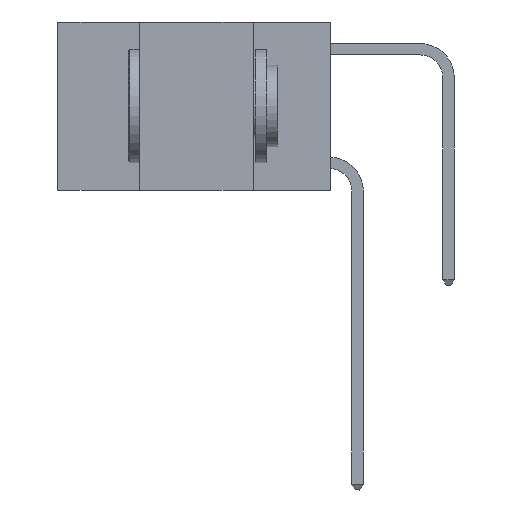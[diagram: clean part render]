
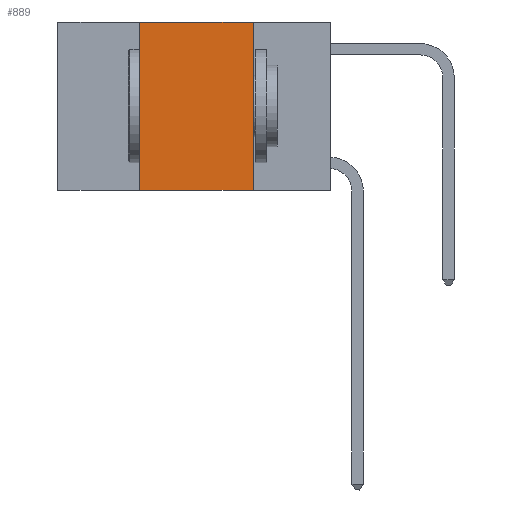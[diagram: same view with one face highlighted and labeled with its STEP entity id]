
A CAD part, left-side view. The second image highlights one B-rep face of the part: STEP entity #889.
In plain terms, the highlighted planar face has unit normal (-1, 0, 0).
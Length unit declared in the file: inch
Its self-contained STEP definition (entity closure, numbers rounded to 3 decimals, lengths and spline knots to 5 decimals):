
#241 = ORIENTED_EDGE ( 'NONE', *, *, #9986, .F. ) ;
#254 = ORIENTED_EDGE ( 'NONE', *, *, #3844, .F. ) ;
#283 = DIRECTION ( 'NONE',  ( 0., 0., 1. ) ) ;
#298 = ORIENTED_EDGE ( 'NONE', *, *, #2192, .F. ) ;
#307 = ORIENTED_EDGE ( 'NONE', *, *, #10433, .T. ) ;
#889 = ADVANCED_FACE ( 'NONE', ( #7766 ), #7281, .F. ) ;
#1146 = CARTESIAN_POINT ( 'NONE',  ( 0., 0.42, 0. ) ) ;
#1429 = VERTEX_POINT ( 'NONE', #4539 ) ;
#1534 = VERTEX_POINT ( 'NONE', #2577 ) ;
#1878 = AXIS2_PLACEMENT_3D ( 'NONE', #8515, #9444, #8858 ) ;
#1986 = CARTESIAN_POINT ( 'NONE',  ( 0., 0.6, -0.37 ) ) ;
#2105 = LINE ( 'NONE', #1146, #11411 ) ;
#2192 = EDGE_CURVE ( 'NONE', #5058, #8914, #2105, .T. ) ;
#2577 = CARTESIAN_POINT ( 'NONE',  ( 0., 0.17, -0.37 ) ) ;
#3656 = LINE ( 'NONE', #11388, #11294 ) ;
#3844 = EDGE_CURVE ( 'NONE', #8914, #1429, #6991, .T. ) ;
#4204 = LINE ( 'NONE', #1986, #6298 ) ;
#4539 = CARTESIAN_POINT ( 'NONE',  ( 0., 0.17, 0. ) ) ;
#4559 = EDGE_LOOP ( 'NONE', ( #241, #254, #298, #307 ) ) ;
#4565 = CARTESIAN_POINT ( 'NONE',  ( 0., 0.42, -0.37 ) ) ;
#4582 = VECTOR ( 'NONE', #8587, 39.37008 ) ;
#5058 = VERTEX_POINT ( 'NONE', #4565 ) ;
#6082 = DIRECTION ( 'NONE',  ( 0., 0., -1. ) ) ;
#6298 = VECTOR ( 'NONE', #9340, 39.37008 ) ;
#6991 = LINE ( 'NONE', #7652, #4582 ) ;
#7281 = PLANE ( 'NONE',  #1878 ) ;
#7652 = CARTESIAN_POINT ( 'NONE',  ( 0., 0.6, 0. ) ) ;
#7766 = FACE_OUTER_BOUND ( 'NONE', #4559, .T. ) ;
#8112 = CARTESIAN_POINT ( 'NONE',  ( 0., 0.42, 0. ) ) ;
#8515 = CARTESIAN_POINT ( 'NONE',  ( 0., 0.6, 0. ) ) ;
#8587 = DIRECTION ( 'NONE',  ( 0., -1., 0. ) ) ;
#8858 = DIRECTION ( 'NONE',  ( 0., 0., -1. ) ) ;
#8914 = VERTEX_POINT ( 'NONE', #8112 ) ;
#9340 = DIRECTION ( 'NONE',  ( 0., -1., 0. ) ) ;
#9444 = DIRECTION ( 'NONE',  ( 1., 0., 0. ) ) ;
#9986 = EDGE_CURVE ( 'NONE', #1429, #1534, #3656, .T. ) ;
#10433 = EDGE_CURVE ( 'NONE', #5058, #1534, #4204, .T. ) ;
#11294 = VECTOR ( 'NONE', #6082, 39.37008 ) ;
#11388 = CARTESIAN_POINT ( 'NONE',  ( 0., 0.17, 0. ) ) ;
#11411 = VECTOR ( 'NONE', #283, 39.37008 ) ;
